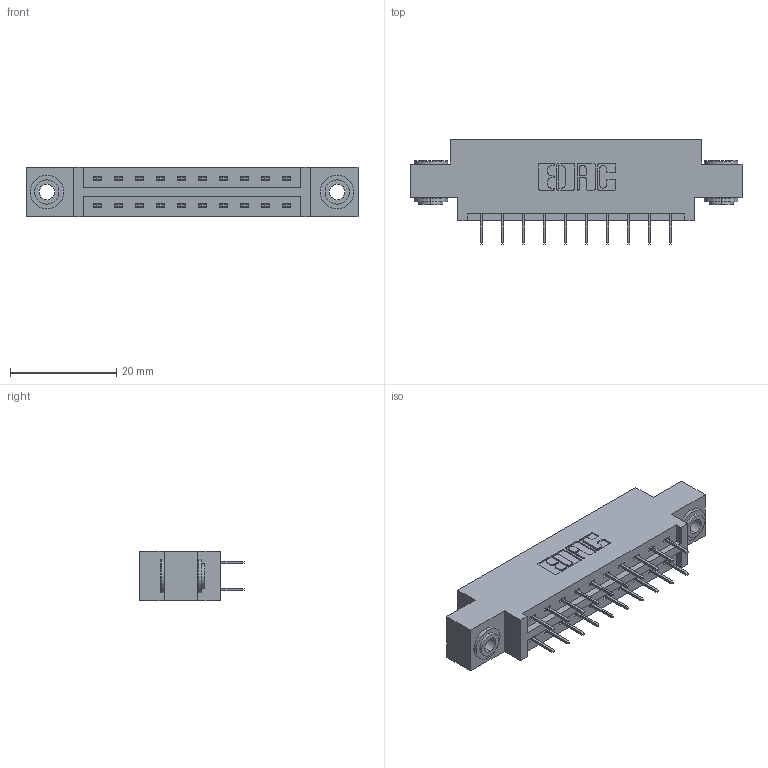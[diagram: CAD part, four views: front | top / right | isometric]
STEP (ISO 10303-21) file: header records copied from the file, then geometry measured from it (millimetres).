
FILE_DESCRIPTION (( 'STEP AP203' ), '1' );
FILE_NAME ('337-020-524-803.STEP', '2018-08-05T08:59:23', ( '' ), ( '' ), 'SwSTEP 2.0', 'SolidWorks 2016', '' );
FILE_SCHEMA (( 'CONFIG_CONTROL_DESIGN' ));
Length unit declared in the file: inch
Products named in the file (4): 337 Part_0.170 Offset - 0.156 Dia-TH; 345-292-001_345-293-124; 345-250-002_345-250-002-102; 337-020-524-803
Assembly tree (23 placements, depth 2):
  337-020-524-803
    337 Part_0.170 Offset - 0.156 Dia-TH
    345-292-001_345-293-124  x20
    345-250-002_345-250-002-102  x2
Bounding box: 62.64 x 19.69 x 9.4 mm (x, y, z)
Volume: 6046.8 mm3; surface area: 6763.6 mm2
Topology: 23 solids, 23 shells, 1316 faces, 3699 edges, 2382 vertices
Faces by surface type: plane 964, cylinder 344, cone 8
Entity records: 12748 total; most frequent: CARTESIAN_POINT 2149, ORIENTED_EDGE 2078, DIRECTION 1921, EDGE_CURVE 1039, LINE 891, VECTOR 891, VERTEX_POINT 686, AXIS2_PLACEMENT_3D 515
